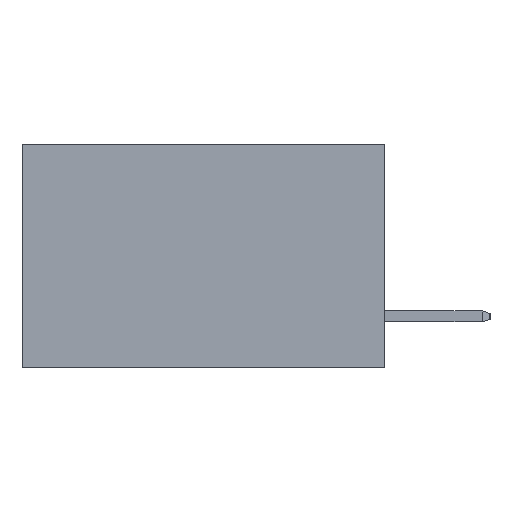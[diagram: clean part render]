
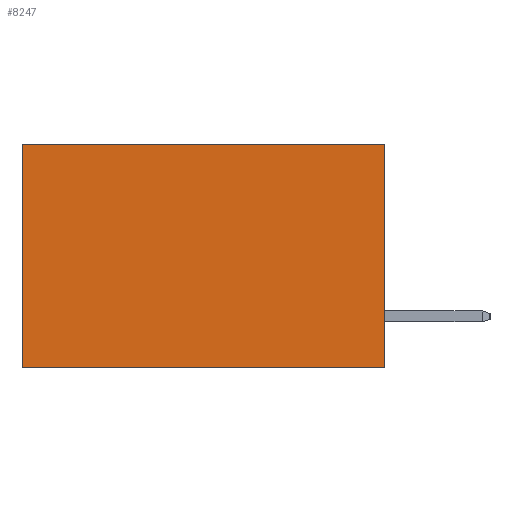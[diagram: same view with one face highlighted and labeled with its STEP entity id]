
A CAD part, left-side view. The second image highlights one B-rep face of the part: STEP entity #8247.
In plain terms, the highlighted planar face has unit normal (-1, 0, 0).
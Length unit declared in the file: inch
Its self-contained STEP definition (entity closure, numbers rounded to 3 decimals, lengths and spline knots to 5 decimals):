
#349 = ORIENTED_EDGE ( 'NONE', *, *, #2511, .T. ) ;
#436 = ORIENTED_EDGE ( 'NONE', *, *, #1175, .F. ) ;
#450 = ORIENTED_EDGE ( 'NONE', *, *, #4189, .F. ) ;
#472 = ORIENTED_EDGE ( 'NONE', *, *, #3431, .T. ) ;
#621 = VERTEX_POINT ( 'NONE', #9135 ) ;
#678 = PLANE ( 'NONE',  #834 ) ;
#834 = AXIS2_PLACEMENT_3D ( 'NONE', #8145, #6560, #1550 ) ;
#902 = CARTESIAN_POINT ( 'NONE',  ( 0.2615, 0., 0. ) ) ;
#1175 = EDGE_CURVE ( 'NONE', #621, #2432, #1256, .T. ) ;
#1256 = LINE ( 'NONE', #6722, #3667 ) ;
#1550 = DIRECTION ( 'NONE',  ( 0., 0., -1. ) ) ;
#2432 = VERTEX_POINT ( 'NONE', #8608 ) ;
#2468 = LINE ( 'NONE', #6395, #6583 ) ;
#2503 = DIRECTION ( 'NONE',  ( 0., 1., 0. ) ) ;
#2511 = EDGE_CURVE ( 'NONE', #621, #6443, #6483, .T. ) ;
#2602 = DIRECTION ( 'NONE',  ( 0., 1., 0. ) ) ;
#3431 = EDGE_CURVE ( 'NONE', #6443, #4788, #6720, .T. ) ;
#3667 = VECTOR ( 'NONE', #7289, 39.37008 ) ;
#4189 = EDGE_CURVE ( 'NONE', #2432, #4788, #2468, .T. ) ;
#4191 = VECTOR ( 'NONE', #2503, 39.37008 ) ;
#4484 = EDGE_LOOP ( 'NONE', ( #472, #450, #436, #349 ) ) ;
#4788 = VERTEX_POINT ( 'NONE', #5975 ) ;
#5975 = CARTESIAN_POINT ( 'NONE',  ( 0.2615, 0.6, -0.37 ) ) ;
#6395 = CARTESIAN_POINT ( 'NONE',  ( 0.2615, 0., -0.37 ) ) ;
#6443 = VERTEX_POINT ( 'NONE', #8836 ) ;
#6483 = LINE ( 'NONE', #902, #4191 ) ;
#6560 = DIRECTION ( 'NONE',  ( 1., 0., 0. ) ) ;
#6583 = VECTOR ( 'NONE', #2602, 39.37008 ) ;
#6720 = LINE ( 'NONE', #9641, #10528 ) ;
#6722 = CARTESIAN_POINT ( 'NONE',  ( 0.2615, 0., -0.37 ) ) ;
#7289 = DIRECTION ( 'NONE',  ( 0., 0., -1. ) ) ;
#8118 = DIRECTION ( 'NONE',  ( 0., 0., -1. ) ) ;
#8145 = CARTESIAN_POINT ( 'NONE',  ( 0.2615, 0., -0.37 ) ) ;
#8247 = ADVANCED_FACE ( 'NONE', ( #9243 ), #678, .F. ) ;
#8608 = CARTESIAN_POINT ( 'NONE',  ( 0.2615, 0., -0.37 ) ) ;
#8836 = CARTESIAN_POINT ( 'NONE',  ( 0.2615, 0.6, 0. ) ) ;
#9135 = CARTESIAN_POINT ( 'NONE',  ( 0.2615, 0., 0. ) ) ;
#9243 = FACE_OUTER_BOUND ( 'NONE', #4484, .T. ) ;
#9641 = CARTESIAN_POINT ( 'NONE',  ( 0.2615, 0.6, -0.37 ) ) ;
#10528 = VECTOR ( 'NONE', #8118, 39.37008 ) ;
